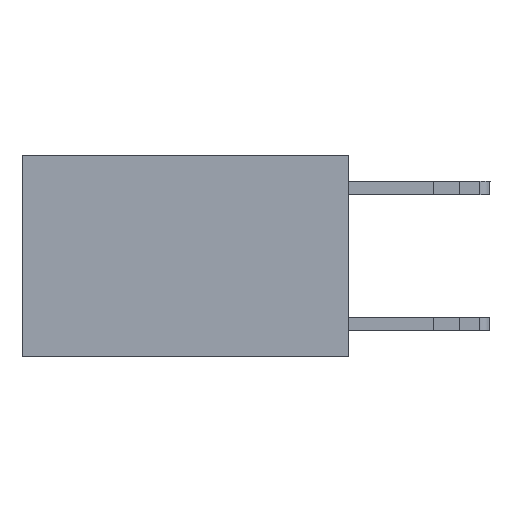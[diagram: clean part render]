
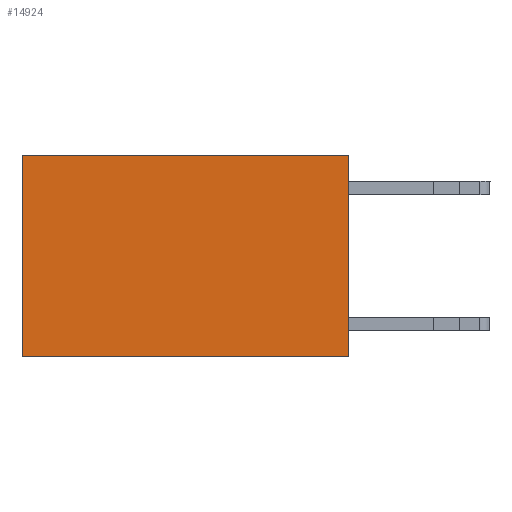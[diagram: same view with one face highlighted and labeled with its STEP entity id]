
A CAD part, left-side view. The second image highlights one B-rep face of the part: STEP entity #14924.
In plain terms, the highlighted planar face has unit normal (-1, 0, 0).
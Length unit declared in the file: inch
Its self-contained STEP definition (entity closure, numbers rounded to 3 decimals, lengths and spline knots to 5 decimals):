
#1034 = CARTESIAN_POINT ( 'NONE',  ( 0.2625, 0., 0. ) ) ;
#1061 = VERTEX_POINT ( 'NONE', #4094 ) ;
#1785 = EDGE_CURVE ( 'NONE', #17769, #7986, #13124, .T. ) ;
#2001 = VECTOR ( 'NONE', #6122, 39.37008 ) ;
#3778 = FACE_OUTER_BOUND ( 'NONE', #18933, .T. ) ;
#4094 = CARTESIAN_POINT ( 'NONE',  ( 0.2625, 0., -0.37 ) ) ;
#4510 = LINE ( 'NONE', #21153, #13098 ) ;
#4559 = EDGE_CURVE ( 'NONE', #17769, #1061, #4510, .T. ) ;
#4649 = CARTESIAN_POINT ( 'NONE',  ( 0.2625, 0.6, -0.37 ) ) ;
#5134 = DIRECTION ( 'NONE',  ( 0., 0., -1. ) ) ;
#6122 = DIRECTION ( 'NONE',  ( 0., 1., 0. ) ) ;
#6952 = VERTEX_POINT ( 'NONE', #4649 ) ;
#7986 = VERTEX_POINT ( 'NONE', #18682 ) ;
#8041 = CARTESIAN_POINT ( 'NONE',  ( 0.2625, 0., -0.37 ) ) ;
#8180 = ORIENTED_EDGE ( 'NONE', *, *, #4559, .F. ) ;
#8398 = ORIENTED_EDGE ( 'NONE', *, *, #1785, .T. ) ;
#8943 = AXIS2_PLACEMENT_3D ( 'NONE', #9003, #15773, #15888 ) ;
#9003 = CARTESIAN_POINT ( 'NONE',  ( 0.2625, 0., 0. ) ) ;
#10265 = ORIENTED_EDGE ( 'NONE', *, *, #15622, .T. ) ;
#11004 = PLANE ( 'NONE',  #8943 ) ;
#11372 = LINE ( 'NONE', #8041, #20494 ) ;
#11700 = DIRECTION ( 'NONE',  ( 0., 1., 0. ) ) ;
#12536 = ORIENTED_EDGE ( 'NONE', *, *, #15437, .F. ) ;
#12867 = CARTESIAN_POINT ( 'NONE',  ( 0.2625, 0., 0. ) ) ;
#13098 = VECTOR ( 'NONE', #14729, 39.37008 ) ;
#13124 = LINE ( 'NONE', #1034, #2001 ) ;
#13908 = LINE ( 'NONE', #20662, #19081 ) ;
#14729 = DIRECTION ( 'NONE',  ( 0., 0., -1. ) ) ;
#14924 = ADVANCED_FACE ( 'NONE', ( #3778 ), #11004, .F. ) ;
#15437 = EDGE_CURVE ( 'NONE', #1061, #6952, #11372, .T. ) ;
#15622 = EDGE_CURVE ( 'NONE', #7986, #6952, #13908, .T. ) ;
#15773 = DIRECTION ( 'NONE',  ( 1., 0., 0. ) ) ;
#15888 = DIRECTION ( 'NONE',  ( 0., 0., -1. ) ) ;
#17769 = VERTEX_POINT ( 'NONE', #12867 ) ;
#18682 = CARTESIAN_POINT ( 'NONE',  ( 0.2625, 0.6, 0. ) ) ;
#18933 = EDGE_LOOP ( 'NONE', ( #10265, #12536, #8180, #8398 ) ) ;
#19081 = VECTOR ( 'NONE', #5134, 39.37008 ) ;
#20494 = VECTOR ( 'NONE', #11700, 39.37008 ) ;
#20662 = CARTESIAN_POINT ( 'NONE',  ( 0.2625, 0.6, 0. ) ) ;
#21153 = CARTESIAN_POINT ( 'NONE',  ( 0.2625, 0., 0. ) ) ;
